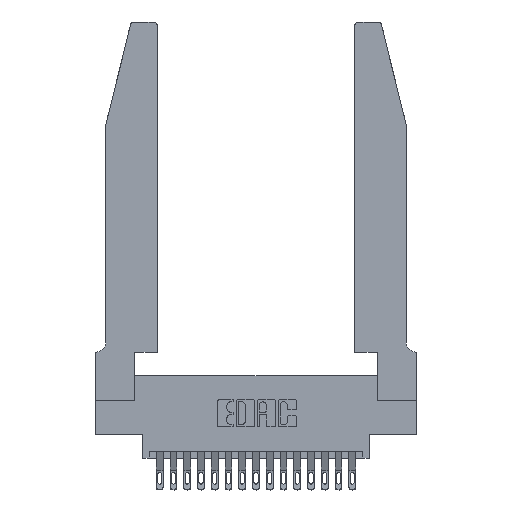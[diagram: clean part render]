
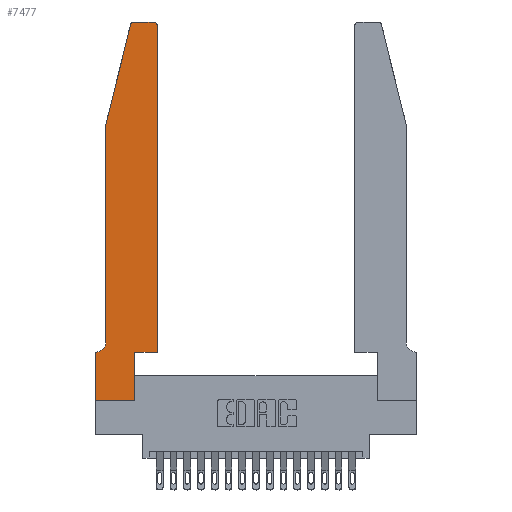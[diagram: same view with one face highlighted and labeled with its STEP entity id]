
A CAD part, top view. The second image highlights one B-rep face of the part: STEP entity #7477.
In plain terms, the highlighted planar face has unit normal (0, 0, 1).
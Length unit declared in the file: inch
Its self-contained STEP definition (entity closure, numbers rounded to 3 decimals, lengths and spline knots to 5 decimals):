
#404 = PLANE ( 'NONE',  #12383 ) ;
#471 = CIRCLE ( 'NONE', #2787, 0.03 ) ;
#850 = ORIENTED_EDGE ( 'NONE', *, *, #14584, .T. ) ;
#1110 = CARTESIAN_POINT ( 'NONE',  ( 0.284, 2.75, 0.37 ) ) ;
#1287 = CARTESIAN_POINT ( 'NONE',  ( 0.0755, 0.42, 0.37 ) ) ;
#1450 = EDGE_CURVE ( 'NONE', #14109, #20055, #1689, .T. ) ;
#1689 = CIRCLE ( 'NONE', #15211, 0.07 ) ;
#1926 = EDGE_CURVE ( 'NONE', #16257, #4795, #16461, .T. ) ;
#1936 = VERTEX_POINT ( 'NONE', #2242 ) ;
#2109 = DIRECTION ( 'NONE',  ( 0., 0., 1. ) ) ;
#2242 = CARTESIAN_POINT ( 'NONE',  ( 0., 0., 0.37 ) ) ;
#2358 = VECTOR ( 'NONE', #16185, 39.37008 ) ;
#2517 = CARTESIAN_POINT ( 'NONE',  ( 0.4505, 0.35, 0.37 ) ) ;
#2608 = CARTESIAN_POINT ( 'NONE',  ( 0.284, 2.72, 0.37 ) ) ;
#2702 = FACE_OUTER_BOUND ( 'NONE', #3313, .T. ) ;
#2786 = ORIENTED_EDGE ( 'NONE', *, *, #9260, .T. ) ;
#2787 = AXIS2_PLACEMENT_3D ( 'NONE', #2898, #14169, #4574 ) ;
#2802 = DIRECTION ( 'NONE',  ( 0., 1., 0. ) ) ;
#2892 = CARTESIAN_POINT ( 'NONE',  ( 0.0055, 0.35, 0.37 ) ) ;
#2898 = CARTESIAN_POINT ( 'NONE',  ( 0.4205, 2.72, 0.37 ) ) ;
#2900 = EDGE_CURVE ( 'NONE', #8683, #1936, #15948, .T. ) ;
#3201 = ORIENTED_EDGE ( 'NONE', *, *, #1450, .T. ) ;
#3313 = EDGE_LOOP ( 'NONE', ( #13662, #8095, #2786, #7485, #3201, #7713, #3410, #11307, #7264, #11365, #4926, #850 ) ) ;
#3410 = ORIENTED_EDGE ( 'NONE', *, *, #2900, .T. ) ;
#3494 = LINE ( 'NONE', #16953, #15255 ) ;
#4294 = DIRECTION ( 'NONE',  ( 1., 0., 0. ) ) ;
#4352 = VECTOR ( 'NONE', #7671, 39.37008 ) ;
#4574 = DIRECTION ( 'NONE',  ( 1., 0., 0. ) ) ;
#4795 = VERTEX_POINT ( 'NONE', #13249 ) ;
#4926 = ORIENTED_EDGE ( 'NONE', *, *, #1926, .T. ) ;
#5288 = CARTESIAN_POINT ( 'NONE',  ( 0.25487, 2.72718, 0.37 ) ) ;
#6428 = EDGE_CURVE ( 'NONE', #1936, #15398, #3494, .T. ) ;
#6816 = CARTESIAN_POINT ( 'NONE',  ( 0.0755, 2., 0.37 ) ) ;
#6934 = DIRECTION ( 'NONE',  ( 0., 1., 0. ) ) ;
#6976 = LINE ( 'NONE', #19360, #11236 ) ;
#7058 = CIRCLE ( 'NONE', #15013, 0.03 ) ;
#7264 = ORIENTED_EDGE ( 'NONE', *, *, #17023, .T. ) ;
#7477 = ADVANCED_FACE ( 'NONE', ( #2702 ), #404, .T. ) ;
#7485 = ORIENTED_EDGE ( 'NONE', *, *, #16946, .T. ) ;
#7646 = DIRECTION ( 'NONE',  ( 1., 0., 0. ) ) ;
#7671 = DIRECTION ( 'NONE',  ( -1., 0., 0. ) ) ;
#7713 = ORIENTED_EDGE ( 'NONE', *, *, #17162, .T. ) ;
#7816 = DIRECTION ( 'NONE',  ( 1., 0., 0. ) ) ;
#7993 = VERTEX_POINT ( 'NONE', #17754 ) ;
#8095 = ORIENTED_EDGE ( 'NONE', *, *, #14475, .T. ) ;
#8193 = CARTESIAN_POINT ( 'NONE',  ( 0., 0., 0.37 ) ) ;
#8324 = VECTOR ( 'NONE', #10498, 39.37008 ) ;
#8461 = CARTESIAN_POINT ( 'NONE',  ( 0.0755, 2., 0.37 ) ) ;
#8545 = LINE ( 'NONE', #8461, #16748 ) ;
#8683 = VERTEX_POINT ( 'NONE', #12821 ) ;
#8931 = CARTESIAN_POINT ( 'NONE',  ( 0.2605, 2.75, 0.37 ) ) ;
#9260 = EDGE_CURVE ( 'NONE', #12968, #20468, #15182, .T. ) ;
#9369 = CARTESIAN_POINT ( 'NONE',  ( 0.4505, 0.35, 0.37 ) ) ;
#9731 = DIRECTION ( 'NONE',  ( 0., -1., 0. ) ) ;
#9807 = CARTESIAN_POINT ( 'NONE',  ( 0.2865, 0., 0.37 ) ) ;
#10498 = DIRECTION ( 'NONE',  ( -1., 0., 0. ) ) ;
#11013 = CARTESIAN_POINT ( 'NONE',  ( 0.4505, 0.35, 0.37 ) ) ;
#11236 = VECTOR ( 'NONE', #6934, 39.37008 ) ;
#11307 = ORIENTED_EDGE ( 'NONE', *, *, #6428, .T. ) ;
#11365 = ORIENTED_EDGE ( 'NONE', *, *, #13374, .T. ) ;
#11723 = DIRECTION ( 'NONE',  ( 0., 0., -1. ) ) ;
#11882 = VECTOR ( 'NONE', #9731, 39.37008 ) ;
#12383 = AXIS2_PLACEMENT_3D ( 'NONE', #13385, #2109, #13455 ) ;
#12613 = CARTESIAN_POINT ( 'NONE',  ( 0.2865, 0.35, 0.37 ) ) ;
#12821 = CARTESIAN_POINT ( 'NONE',  ( 0., 0.35, 0.37 ) ) ;
#12968 = VERTEX_POINT ( 'NONE', #5288 ) ;
#13249 = CARTESIAN_POINT ( 'NONE',  ( 0.4505, 2.72, 0.37 ) ) ;
#13374 = EDGE_CURVE ( 'NONE', #17951, #16257, #16146, .T. ) ;
#13385 = CARTESIAN_POINT ( 'NONE',  ( 0., 0.35, 0.37 ) ) ;
#13455 = DIRECTION ( 'NONE',  ( 1., 0., 0. ) ) ;
#13662 = ORIENTED_EDGE ( 'NONE', *, *, #15053, .T. ) ;
#13913 = DIRECTION ( 'NONE',  ( 0., 0., 1. ) ) ;
#14109 = VERTEX_POINT ( 'NONE', #1287 ) ;
#14169 = DIRECTION ( 'NONE',  ( 0., 0., 1. ) ) ;
#14475 = EDGE_CURVE ( 'NONE', #20041, #12968, #7058, .T. ) ;
#14584 = EDGE_CURVE ( 'NONE', #4795, #7993, #471, .T. ) ;
#15013 = AXIS2_PLACEMENT_3D ( 'NONE', #2608, #13913, #4294 ) ;
#15053 = EDGE_CURVE ( 'NONE', #7993, #20041, #20618, .T. ) ;
#15182 = LINE ( 'NONE', #6816, #2358 ) ;
#15211 = AXIS2_PLACEMENT_3D ( 'NONE', #18919, #11723, #20053 ) ;
#15255 = VECTOR ( 'NONE', #7646, 39.37008 ) ;
#15398 = VERTEX_POINT ( 'NONE', #9807 ) ;
#15678 = VECTOR ( 'NONE', #7816, 39.37008 ) ;
#15948 = LINE ( 'NONE', #8193, #11882 ) ;
#16146 = LINE ( 'NONE', #11013, #15678 ) ;
#16185 = DIRECTION ( 'NONE',  ( -0.239, -0.971, 0. ) ) ;
#16257 = VERTEX_POINT ( 'NONE', #9369 ) ;
#16461 = LINE ( 'NONE', #2517, #19550 ) ;
#16748 = VECTOR ( 'NONE', #17704, 39.37008 ) ;
#16946 = EDGE_CURVE ( 'NONE', #20468, #14109, #8545, .T. ) ;
#16953 = CARTESIAN_POINT ( 'NONE',  ( 0., 0., 0.37 ) ) ;
#17023 = EDGE_CURVE ( 'NONE', #15398, #17951, #6976, .T. ) ;
#17162 = EDGE_CURVE ( 'NONE', #20055, #8683, #20566, .T. ) ;
#17704 = DIRECTION ( 'NONE',  ( 0., -1., 0. ) ) ;
#17754 = CARTESIAN_POINT ( 'NONE',  ( 0.4205, 2.75, 0.37 ) ) ;
#17951 = VERTEX_POINT ( 'NONE', #12613 ) ;
#18136 = CARTESIAN_POINT ( 'NONE',  ( 0.0755, 2., 0.37 ) ) ;
#18495 = CARTESIAN_POINT ( 'NONE',  ( 0.0755, 0.35, 0.37 ) ) ;
#18919 = CARTESIAN_POINT ( 'NONE',  ( 0.0055, 0.42, 0.37 ) ) ;
#19360 = CARTESIAN_POINT ( 'NONE',  ( 0.2865, 0.35, 0.37 ) ) ;
#19550 = VECTOR ( 'NONE', #2802, 39.37008 ) ;
#20041 = VERTEX_POINT ( 'NONE', #1110 ) ;
#20053 = DIRECTION ( 'NONE',  ( -1., 0., 0. ) ) ;
#20055 = VERTEX_POINT ( 'NONE', #2892 ) ;
#20468 = VERTEX_POINT ( 'NONE', #18136 ) ;
#20566 = LINE ( 'NONE', #18495, #4352 ) ;
#20618 = LINE ( 'NONE', #8931, #8324 ) ;
